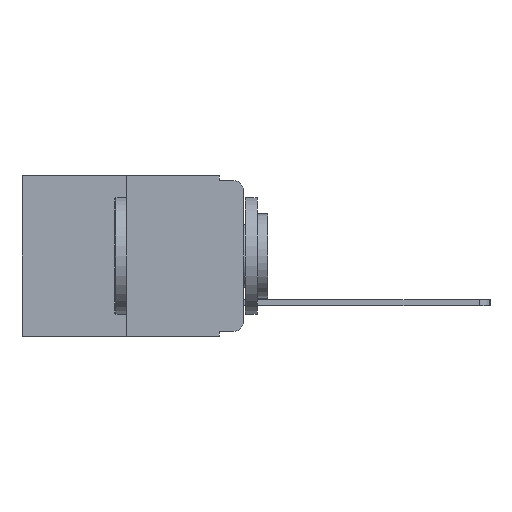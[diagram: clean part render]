
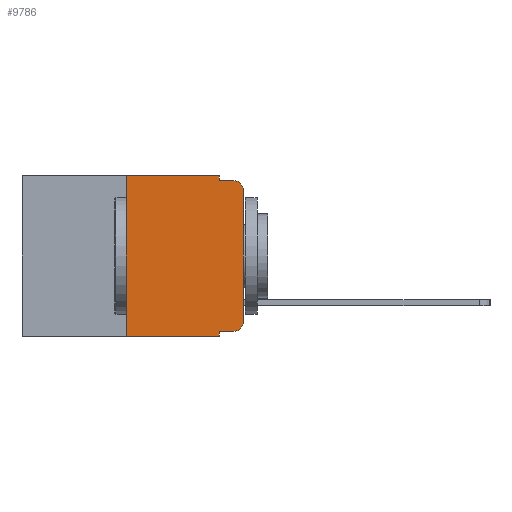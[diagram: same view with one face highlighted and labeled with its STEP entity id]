
A CAD part, left-side view. The second image highlights one B-rep face of the part: STEP entity #9786.
In plain terms, the highlighted planar face has unit normal (-1, 0, 0).
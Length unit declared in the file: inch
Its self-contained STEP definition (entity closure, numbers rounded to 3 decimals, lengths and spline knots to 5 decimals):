
#113 = CARTESIAN_POINT ( 'NONE',  ( 0., 0.051, 0. ) ) ;
#230 = DIRECTION ( 'NONE',  ( -1., 0., 0. ) ) ;
#245 = ORIENTED_EDGE ( 'NONE', *, *, #1919, .T. ) ;
#270 = VECTOR ( 'NONE', #3703, 39.37008 ) ;
#271 = CARTESIAN_POINT ( 'NONE',  ( 0., 0.02, -0.03 ) ) ;
#301 = EDGE_CURVE ( 'NONE', #11298, #5899, #5903, .T. ) ;
#414 = CARTESIAN_POINT ( 'NONE',  ( 0., 0.473, 0. ) ) ;
#432 = DIRECTION ( 'NONE',  ( 0., 0., -1. ) ) ;
#465 = ORIENTED_EDGE ( 'NONE', *, *, #13224, .T. ) ;
#466 = DIRECTION ( 'NONE',  ( 0., 0., -1. ) ) ;
#485 = CARTESIAN_POINT ( 'NONE',  ( 0., 0.02, -0.333 ) ) ;
#809 = CARTESIAN_POINT ( 'NONE',  ( 0., 0.051, -0.333 ) ) ;
#854 = EDGE_CURVE ( 'NONE', #11298, #9953, #5137, .T. ) ;
#1130 = CARTESIAN_POINT ( 'NONE',  ( 0., 0.051, 0. ) ) ;
#1309 = ORIENTED_EDGE ( 'NONE', *, *, #6602, .T. ) ;
#1403 = EDGE_CURVE ( 'NONE', #12737, #2725, #6728, .T. ) ;
#1511 = ORIENTED_EDGE ( 'NONE', *, *, #8028, .F. ) ;
#1512 = ORIENTED_EDGE ( 'NONE', *, *, #3048, .T. ) ;
#1823 = VECTOR ( 'NONE', #6227, 39.37008 ) ;
#1919 = EDGE_CURVE ( 'NONE', #3661, #2725, #6715, .T. ) ;
#2162 = EDGE_LOOP ( 'NONE', ( #1512, #245, #8244, #4126, #1511, #10125, #7388, #7560, #465, #1309 ) ) ;
#2290 = DIRECTION ( 'NONE',  ( 0., -1., 0. ) ) ;
#2291 = FACE_OUTER_BOUND ( 'NONE', #2162, .T. ) ;
#2605 = LINE ( 'NONE', #4802, #13368 ) ;
#2725 = VERTEX_POINT ( 'NONE', #12378 ) ;
#2785 = CARTESIAN_POINT ( 'NONE',  ( 0., 0.051, -0.01 ) ) ;
#2878 = VECTOR ( 'NONE', #5484, 39.37008 ) ;
#3048 = EDGE_CURVE ( 'NONE', #3095, #3661, #12008, .T. ) ;
#3095 = VERTEX_POINT ( 'NONE', #9012 ) ;
#3491 = CARTESIAN_POINT ( 'NONE',  ( 0., 0.25, 0. ) ) ;
#3557 = VECTOR ( 'NONE', #4000, 39.37008 ) ;
#3661 = VERTEX_POINT ( 'NONE', #9929 ) ;
#3703 = DIRECTION ( 'NONE',  ( 0., 0., 1. ) ) ;
#3726 = AXIS2_PLACEMENT_3D ( 'NONE', #271, #230, #432 ) ;
#3744 = EDGE_CURVE ( 'NONE', #11454, #12737, #6169, .T. ) ;
#3785 = VECTOR ( 'NONE', #2290, 39.37008 ) ;
#3807 = VERTEX_POINT ( 'NONE', #485 ) ;
#3913 = CARTESIAN_POINT ( 'NONE',  ( 0., 0.051, -0.01 ) ) ;
#4000 = DIRECTION ( 'NONE',  ( 0., 0., -1. ) ) ;
#4126 = ORIENTED_EDGE ( 'NONE', *, *, #3744, .F. ) ;
#4487 = DIRECTION ( 'NONE',  ( 0., 0., 1. ) ) ;
#4802 = CARTESIAN_POINT ( 'NONE',  ( 0., 0.051, -0.333 ) ) ;
#4922 = EDGE_CURVE ( 'NONE', #12898, #9953, #10609, .T. ) ;
#4978 = PLANE ( 'NONE',  #11646 ) ;
#5137 = LINE ( 'NONE', #7489, #1823 ) ;
#5199 = AXIS2_PLACEMENT_3D ( 'NONE', #12518, #6174, #13538 ) ;
#5355 = CARTESIAN_POINT ( 'NONE',  ( 0., 0.051, -0.343 ) ) ;
#5484 = DIRECTION ( 'NONE',  ( 0., -1., 0. ) ) ;
#5899 = VERTEX_POINT ( 'NONE', #10323 ) ;
#5903 = LINE ( 'NONE', #3491, #11240 ) ;
#6169 = LINE ( 'NONE', #7659, #3557 ) ;
#6174 = DIRECTION ( 'NONE',  ( -1., 0., 0. ) ) ;
#6227 = DIRECTION ( 'NONE',  ( 0., -1., 0. ) ) ;
#6602 = EDGE_CURVE ( 'NONE', #3807, #3095, #7279, .T. ) ;
#6715 = CIRCLE ( 'NONE', #3726, 0.02 ) ;
#6728 = LINE ( 'NONE', #2785, #3785 ) ;
#6939 = CARTESIAN_POINT ( 'NONE',  ( 0., 0., 0. ) ) ;
#7279 = CIRCLE ( 'NONE', #5199, 0.02 ) ;
#7284 = DIRECTION ( 'NONE',  ( 1., 0., 0. ) ) ;
#7388 = ORIENTED_EDGE ( 'NONE', *, *, #854, .T. ) ;
#7489 = CARTESIAN_POINT ( 'NONE',  ( 0., 0.473, -0.343 ) ) ;
#7560 = ORIENTED_EDGE ( 'NONE', *, *, #4922, .F. ) ;
#7659 = CARTESIAN_POINT ( 'NONE',  ( 0., 0.051, 0. ) ) ;
#8028 = EDGE_CURVE ( 'NONE', #5899, #11454, #8395, .T. ) ;
#8134 = DIRECTION ( 'NONE',  ( 0., -1., 0. ) ) ;
#8244 = ORIENTED_EDGE ( 'NONE', *, *, #1403, .F. ) ;
#8395 = LINE ( 'NONE', #13941, #2878 ) ;
#9012 = CARTESIAN_POINT ( 'NONE',  ( 0., 0., -0.313 ) ) ;
#9121 = DIRECTION ( 'NONE',  ( 0., 0., -1. ) ) ;
#9786 = ADVANCED_FACE ( 'NONE', ( #2291 ), #4978, .F. ) ;
#9821 = CARTESIAN_POINT ( 'NONE',  ( 0., 0.25, -0.343 ) ) ;
#9929 = CARTESIAN_POINT ( 'NONE',  ( 0., 0., -0.03 ) ) ;
#9953 = VERTEX_POINT ( 'NONE', #5355 ) ;
#10125 = ORIENTED_EDGE ( 'NONE', *, *, #301, .F. ) ;
#10323 = CARTESIAN_POINT ( 'NONE',  ( 0., 0.25, 0. ) ) ;
#10609 = LINE ( 'NONE', #1130, #13070 ) ;
#11240 = VECTOR ( 'NONE', #4487, 39.37008 ) ;
#11298 = VERTEX_POINT ( 'NONE', #9821 ) ;
#11454 = VERTEX_POINT ( 'NONE', #113 ) ;
#11646 = AXIS2_PLACEMENT_3D ( 'NONE', #414, #7284, #466 ) ;
#12008 = LINE ( 'NONE', #6939, #270 ) ;
#12378 = CARTESIAN_POINT ( 'NONE',  ( 0., 0.02, -0.01 ) ) ;
#12518 = CARTESIAN_POINT ( 'NONE',  ( 0., 0.02, -0.313 ) ) ;
#12737 = VERTEX_POINT ( 'NONE', #3913 ) ;
#12898 = VERTEX_POINT ( 'NONE', #809 ) ;
#13070 = VECTOR ( 'NONE', #9121, 39.37008 ) ;
#13224 = EDGE_CURVE ( 'NONE', #12898, #3807, #2605, .T. ) ;
#13368 = VECTOR ( 'NONE', #8134, 39.37008 ) ;
#13538 = DIRECTION ( 'NONE',  ( 0., 0., -1. ) ) ;
#13941 = CARTESIAN_POINT ( 'NONE',  ( 0., 0.473, 0. ) ) ;
